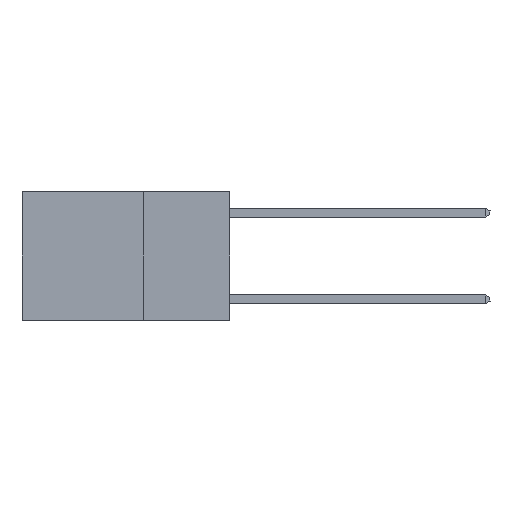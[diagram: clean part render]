
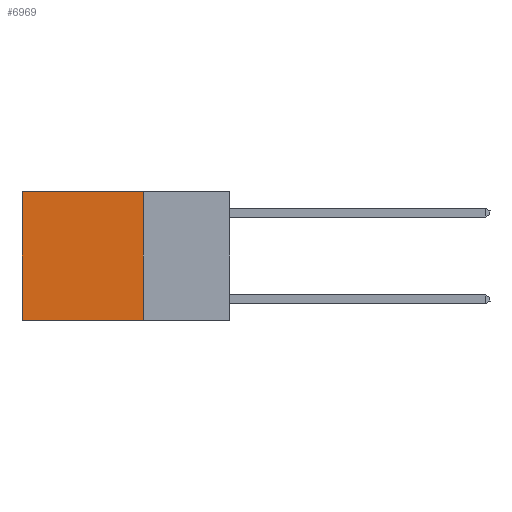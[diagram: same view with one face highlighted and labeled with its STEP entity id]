
A CAD part, left-side view. The second image highlights one B-rep face of the part: STEP entity #6969.
In plain terms, the highlighted planar face has unit normal (-1, 0, 0).
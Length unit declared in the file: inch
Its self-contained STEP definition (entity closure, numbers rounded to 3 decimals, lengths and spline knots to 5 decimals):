
#671 = EDGE_CURVE ( 'NONE', #10548, #3122, #7254, .T. ) ;
#687 = VECTOR ( 'NONE', #17526, 39.37008 ) ;
#1553 = ORIENTED_EDGE ( 'NONE', *, *, #671, .T. ) ;
#2708 = EDGE_CURVE ( 'NONE', #4099, #3122, #8664, .T. ) ;
#2879 = CARTESIAN_POINT ( 'NONE',  ( 0.2625, 0.25, 0. ) ) ;
#3122 = VERTEX_POINT ( 'NONE', #9685 ) ;
#4099 = VERTEX_POINT ( 'NONE', #12907 ) ;
#6080 = DIRECTION ( 'NONE',  ( 0., 1., 0. ) ) ;
#6867 = EDGE_LOOP ( 'NONE', ( #1553, #13371, #11317, #10332 ) ) ;
#6969 = ADVANCED_FACE ( 'NONE', ( #7999 ), #10865, .F. ) ;
#7028 = DIRECTION ( 'NONE',  ( 0., 1., 0. ) ) ;
#7254 = LINE ( 'NONE', #10302, #15078 ) ;
#7525 = CARTESIAN_POINT ( 'NONE',  ( 0.2625, 0.25, 0. ) ) ;
#7999 = FACE_OUTER_BOUND ( 'NONE', #6867, .T. ) ;
#8408 = VECTOR ( 'NONE', #7028, 39.37008 ) ;
#8574 = CARTESIAN_POINT ( 'NONE',  ( 0.2625, 0.25, -0.37 ) ) ;
#8664 = LINE ( 'NONE', #8574, #8408 ) ;
#8789 = DIRECTION ( 'NONE',  ( 0., 0., -1. ) ) ;
#8960 = LINE ( 'NONE', #7525, #14274 ) ;
#9327 = CARTESIAN_POINT ( 'NONE',  ( 0.2625, 0.25, 0. ) ) ;
#9685 = CARTESIAN_POINT ( 'NONE',  ( 0.2625, 0.6, -0.37 ) ) ;
#9690 = AXIS2_PLACEMENT_3D ( 'NONE', #9327, #12421, #10760 ) ;
#10302 = CARTESIAN_POINT ( 'NONE',  ( 0.2625, 0.6, 0. ) ) ;
#10332 = ORIENTED_EDGE ( 'NONE', *, *, #17541, .T. ) ;
#10548 = VERTEX_POINT ( 'NONE', #15711 ) ;
#10760 = DIRECTION ( 'NONE',  ( 0., 0., -1. ) ) ;
#10865 = PLANE ( 'NONE',  #9690 ) ;
#10975 = EDGE_CURVE ( 'NONE', #16010, #4099, #13234, .T. ) ;
#11317 = ORIENTED_EDGE ( 'NONE', *, *, #10975, .F. ) ;
#11618 = CARTESIAN_POINT ( 'NONE',  ( 0.2625, 0.25, 0. ) ) ;
#12421 = DIRECTION ( 'NONE',  ( 1., 0., 0. ) ) ;
#12907 = CARTESIAN_POINT ( 'NONE',  ( 0.2625, 0.25, -0.37 ) ) ;
#13234 = LINE ( 'NONE', #11618, #687 ) ;
#13371 = ORIENTED_EDGE ( 'NONE', *, *, #2708, .F. ) ;
#14274 = VECTOR ( 'NONE', #6080, 39.37008 ) ;
#15078 = VECTOR ( 'NONE', #8789, 39.37008 ) ;
#15711 = CARTESIAN_POINT ( 'NONE',  ( 0.2625, 0.6, 0. ) ) ;
#16010 = VERTEX_POINT ( 'NONE', #2879 ) ;
#17526 = DIRECTION ( 'NONE',  ( 0., 0., -1. ) ) ;
#17541 = EDGE_CURVE ( 'NONE', #16010, #10548, #8960, .T. ) ;
